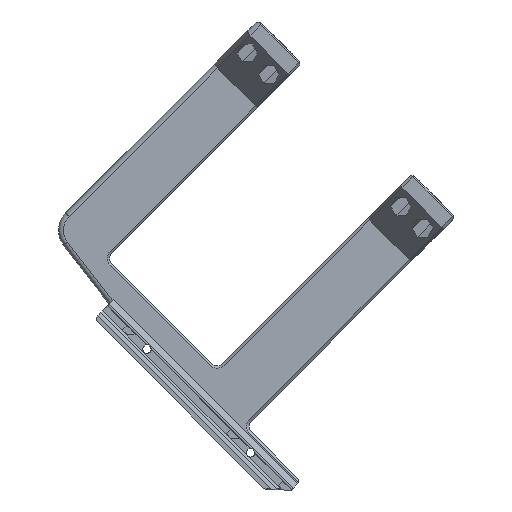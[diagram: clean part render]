
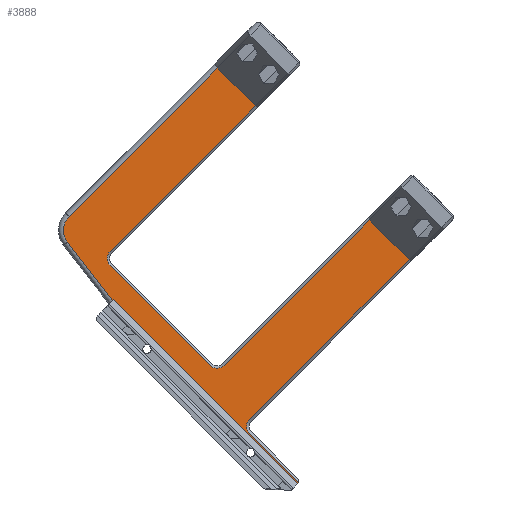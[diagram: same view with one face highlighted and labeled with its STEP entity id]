
A CAD part, left-side view. The second image highlights one B-rep face of the part: STEP entity #3888.
In plain terms, the highlighted planar face has unit normal (-1, 0, 0).
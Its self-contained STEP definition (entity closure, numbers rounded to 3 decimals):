
#130=CIRCLE('',#4140,8.);
#132=CIRCLE('',#4148,4.);
#133=CIRCLE('',#4149,4.);
#134=CIRCLE('',#4150,4.);
#197=FACE_OUTER_BOUND('',#414,.T.);
#414=EDGE_LOOP('',(#2726,#2727,#2728,#2729,#2730,#2731,#2732,#2733,#2734,
#2735,#2736,#2737,#2738,#2739,#2740,#2741));
#673=LINE('',#5632,#1135);
#684=LINE('',#5664,#1146);
#721=LINE('',#5744,#1183);
#722=LINE('',#5756,#1184);
#726=LINE('',#5773,#1188);
#727=LINE('',#5775,#1189);
#728=LINE('',#5779,#1190);
#729=LINE('',#5781,#1191);
#730=LINE('',#5783,#1192);
#731=LINE('',#5787,#1193);
#732=LINE('',#5791,#1194);
#733=LINE('',#5792,#1195);
#1135=VECTOR('',#4490,10.);
#1146=VECTOR('',#4505,10.);
#1183=VECTOR('',#4568,10.);
#1184=VECTOR('',#4585,10.);
#1188=VECTOR('',#4597,10.);
#1189=VECTOR('',#4598,10.);
#1190=VECTOR('',#4601,10.);
#1191=VECTOR('',#4602,10.);
#1192=VECTOR('',#4603,10.);
#1193=VECTOR('',#4606,10.);
#1194=VECTOR('',#4609,10.);
#1195=VECTOR('',#4610,10.);
#1648=VERTEX_POINT('',#5629);
#1649=VERTEX_POINT('',#5631);
#1660=VERTEX_POINT('',#5662);
#1689=VERTEX_POINT('',#5742);
#1690=VERTEX_POINT('',#5743);
#1691=VERTEX_POINT('',#5748);
#1696=VERTEX_POINT('',#5772);
#1697=VERTEX_POINT('',#5774);
#1698=VERTEX_POINT('',#5776);
#1699=VERTEX_POINT('',#5778);
#1700=VERTEX_POINT('',#5780);
#1701=VERTEX_POINT('',#5782);
#1702=VERTEX_POINT('',#5784);
#1703=VERTEX_POINT('',#5786);
#1704=VERTEX_POINT('',#5788);
#1705=VERTEX_POINT('',#5790);
#2032=EDGE_CURVE('',#1649,#1648,#673,.T.);
#2045=EDGE_CURVE('',#1660,#1648,#684,.F.);
#2084=EDGE_CURVE('',#1689,#1690,#721,.T.);
#2088=EDGE_CURVE('',#1690,#1691,#130,.T.);
#2091=EDGE_CURVE('',#1691,#1649,#722,.T.);
#2097=EDGE_CURVE('',#1660,#1696,#726,.T.);
#2098=EDGE_CURVE('',#1696,#1697,#727,.T.);
#2099=EDGE_CURVE('',#1697,#1698,#132,.T.);
#2100=EDGE_CURVE('',#1698,#1699,#728,.T.);
#2101=EDGE_CURVE('',#1700,#1699,#729,.T.);
#2102=EDGE_CURVE('',#1700,#1701,#730,.T.);
#2103=EDGE_CURVE('',#1701,#1702,#133,.T.);
#2104=EDGE_CURVE('',#1702,#1703,#731,.T.);
#2105=EDGE_CURVE('',#1703,#1704,#134,.T.);
#2106=EDGE_CURVE('',#1704,#1705,#732,.T.);
#2107=EDGE_CURVE('',#1689,#1705,#733,.T.);
#2726=ORIENTED_EDGE('',*,*,#2091,.T.);
#2727=ORIENTED_EDGE('',*,*,#2032,.T.);
#2728=ORIENTED_EDGE('',*,*,#2045,.F.);
#2729=ORIENTED_EDGE('',*,*,#2097,.T.);
#2730=ORIENTED_EDGE('',*,*,#2098,.T.);
#2731=ORIENTED_EDGE('',*,*,#2099,.T.);
#2732=ORIENTED_EDGE('',*,*,#2100,.T.);
#2733=ORIENTED_EDGE('',*,*,#2101,.F.);
#2734=ORIENTED_EDGE('',*,*,#2102,.T.);
#2735=ORIENTED_EDGE('',*,*,#2103,.T.);
#2736=ORIENTED_EDGE('',*,*,#2104,.T.);
#2737=ORIENTED_EDGE('',*,*,#2105,.T.);
#2738=ORIENTED_EDGE('',*,*,#2106,.T.);
#2739=ORIENTED_EDGE('',*,*,#2107,.F.);
#2740=ORIENTED_EDGE('',*,*,#2084,.T.);
#2741=ORIENTED_EDGE('',*,*,#2088,.T.);
#3712=PLANE('',#4147);
#3888=ADVANCED_FACE('',(#197),#3712,.F.);
#4140=AXIS2_PLACEMENT_3D('',#5751,#4577,#4578);
#4147=AXIS2_PLACEMENT_3D('',#5771,#4595,#4596);
#4148=AXIS2_PLACEMENT_3D('',#5777,#4599,#4600);
#4149=AXIS2_PLACEMENT_3D('',#5785,#4604,#4605);
#4150=AXIS2_PLACEMENT_3D('',#5789,#4607,#4608);
#4490=DIRECTION('',(0.,-0.707,0.707));
#4505=DIRECTION('',(0.,-0.707,-0.707));
#4568=DIRECTION('',(0.,0.707,-0.707));
#4577=DIRECTION('center_axis',(-1.,0.,0.));
#4578=DIRECTION('ref_axis',(0.,0.998,0.064));
#4585=DIRECTION('',(0.,-0.611,-0.791));
#4595=DIRECTION('center_axis',(1.,0.,0.));
#4596=DIRECTION('ref_axis',(0.,0.707,0.707));
#4597=DIRECTION('',(0.,-0.707,0.707));
#4598=DIRECTION('',(0.,0.707,0.707));
#4599=DIRECTION('center_axis',(1.,0.,0.));
#4600=DIRECTION('ref_axis',(0.,1.,0.));
#4601=DIRECTION('',(0.,-0.707,0.707));
#4602=DIRECTION('',(0.,-0.707,-0.707));
#4603=DIRECTION('',(0.,0.707,-0.707));
#4604=DIRECTION('center_axis',(1.,0.,0.));
#4605=DIRECTION('ref_axis',(0.,0.,-1.));
#4606=DIRECTION('',(0.,0.707,0.707));
#4607=DIRECTION('center_axis',(1.,0.,0.));
#4608=DIRECTION('ref_axis',(0.,1.,0.));
#4609=DIRECTION('',(0.,-0.707,0.707));
#4610=DIRECTION('',(0.,-0.707,-0.707));
#5629=CARTESIAN_POINT('',(-8.23,90.288,80.498));
#5631=CARTESIAN_POINT('',(-8.23,90.707,80.078));
#5632=CARTESIAN_POINT('',(-8.23,91.425,79.361));
#5662=CARTESIAN_POINT('',(-8.23,14.91,5.12));
#5664=CARTESIAN_POINT('',(-8.23,24.173,14.384));
#5742=CARTESIAN_POINT('',(-8.23,47.776,175.336));
#5743=CARTESIAN_POINT('',(-8.23,108.538,114.574));
#5744=CARTESIAN_POINT('',(-8.23,115.336,107.775));
#5748=CARTESIAN_POINT('',(-8.23,109.211,104.025));
#5751=CARTESIAN_POINT('Origin',(-8.23,102.881,108.917));
#5756=CARTESIAN_POINT('',(-8.23,73.982,58.433));
#5771=CARTESIAN_POINT('Origin',(-8.23,36.14,28.579));
#5772=CARTESIAN_POINT('',(-8.23,14.503,5.528));
#5773=CARTESIAN_POINT('',(-8.23,-4.767,24.798));
#5774=CARTESIAN_POINT('',(-8.23,34.726,25.751));
#5775=CARTESIAN_POINT('',(-8.23,23.766,14.791));
#5776=CARTESIAN_POINT('',(-8.23,34.726,31.408));
#5777=CARTESIAN_POINT('Origin',(-8.23,31.898,28.579));
#5778=CARTESIAN_POINT('',(-8.23,-30.713,96.847));
#5779=CARTESIAN_POINT('',(-8.23,36.848,29.286));
#5780=CARTESIAN_POINT('',(-8.23,-14.449,113.11));
#5781=CARTESIAN_POINT('',(-8.23,-31.42,96.14));
#5782=CARTESIAN_POINT('',(-8.23,45.11,53.551));
#5783=CARTESIAN_POINT('',(-8.23,26.483,72.178));
#5784=CARTESIAN_POINT('',(-8.23,50.767,53.551));
#5785=CARTESIAN_POINT('Origin',(-8.23,47.939,56.379));
#5786=CARTESIAN_POINT('',(-8.23,91.779,94.563));
#5787=CARTESIAN_POINT('',(-8.23,51.121,53.904));
#5788=CARTESIAN_POINT('',(-8.23,91.779,100.22));
#5789=CARTESIAN_POINT('Origin',(-8.23,88.951,97.391));
#5790=CARTESIAN_POINT('',(-8.23,32.22,159.779));
#5791=CARTESIAN_POINT('',(-8.23,73.152,118.847));
#5792=CARTESIAN_POINT('',(-8.23,0.046,127.606));
